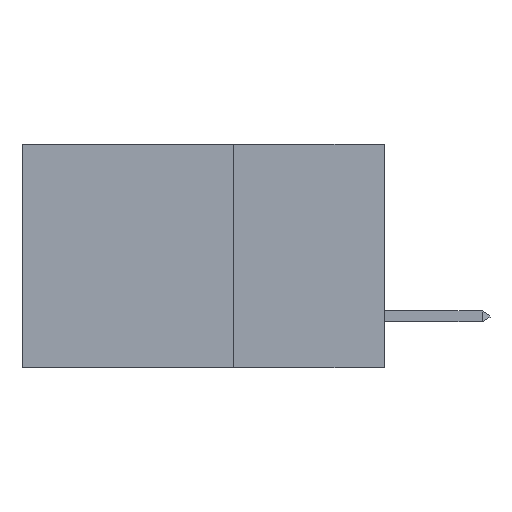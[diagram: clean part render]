
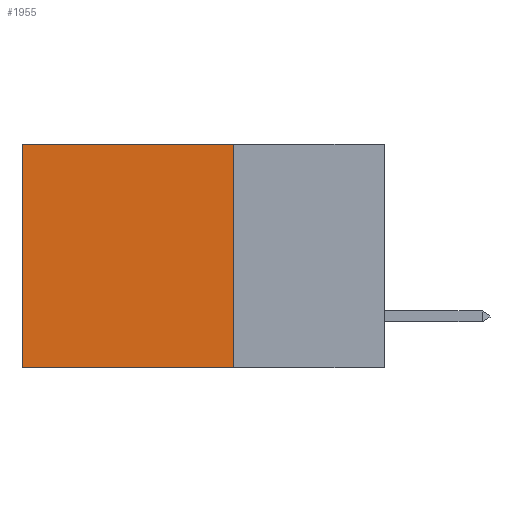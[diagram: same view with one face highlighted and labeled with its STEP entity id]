
A CAD part, left-side view. The second image highlights one B-rep face of the part: STEP entity #1955.
In plain terms, the highlighted planar face has unit normal (-1, 0, 0).
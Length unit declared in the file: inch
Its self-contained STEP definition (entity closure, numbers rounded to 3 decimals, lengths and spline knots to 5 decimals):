
#151 = VERTEX_POINT ( 'NONE', #10503 ) ;
#1612 = CARTESIAN_POINT ( 'NONE',  ( 0.2875, 0.6, 0. ) ) ;
#1689 = LINE ( 'NONE', #12362, #12950 ) ;
#1955 = ADVANCED_FACE ( 'NONE', ( #15050 ), #16464, .F. ) ;
#2047 = CARTESIAN_POINT ( 'NONE',  ( 0.2875, 0.25, -0.37 ) ) ;
#2986 = VERTEX_POINT ( 'NONE', #16378 ) ;
#3120 = DIRECTION ( 'NONE',  ( 0., 0., -1. ) ) ;
#3266 = VECTOR ( 'NONE', #13111, 39.37008 ) ;
#4010 = LINE ( 'NONE', #1612, #14661 ) ;
#4297 = EDGE_CURVE ( 'NONE', #151, #12354, #7303, .T. ) ;
#5060 = DIRECTION ( 'NONE',  ( 0., 1., 0. ) ) ;
#5773 = EDGE_LOOP ( 'NONE', ( #12469, #10964, #14122, #10629 ) ) ;
#6057 = CARTESIAN_POINT ( 'NONE',  ( 0.2875, 0.25, 0. ) ) ;
#7303 = LINE ( 'NONE', #15601, #3266 ) ;
#8840 = EDGE_CURVE ( 'NONE', #2986, #11443, #4010, .T. ) ;
#9416 = DIRECTION ( 'NONE',  ( 0., 0., -1. ) ) ;
#10264 = CARTESIAN_POINT ( 'NONE',  ( 0.2875, 0.6, -0.37 ) ) ;
#10347 = VECTOR ( 'NONE', #17449, 39.37008 ) ;
#10503 = CARTESIAN_POINT ( 'NONE',  ( 0.2875, 0.25, 0. ) ) ;
#10629 = ORIENTED_EDGE ( 'NONE', *, *, #16732, .T. ) ;
#10964 = ORIENTED_EDGE ( 'NONE', *, *, #13193, .F. ) ;
#11443 = VERTEX_POINT ( 'NONE', #10264 ) ;
#12354 = VERTEX_POINT ( 'NONE', #2047 ) ;
#12362 = CARTESIAN_POINT ( 'NONE',  ( 0.2875, 0.25, -0.37 ) ) ;
#12469 = ORIENTED_EDGE ( 'NONE', *, *, #8840, .T. ) ;
#12950 = VECTOR ( 'NONE', #5060, 39.37008 ) ;
#13111 = DIRECTION ( 'NONE',  ( 0., 0., -1. ) ) ;
#13193 = EDGE_CURVE ( 'NONE', #12354, #11443, #1689, .T. ) ;
#13976 = LINE ( 'NONE', #6057, #10347 ) ;
#14122 = ORIENTED_EDGE ( 'NONE', *, *, #4297, .F. ) ;
#14661 = VECTOR ( 'NONE', #3120, 39.37008 ) ;
#15050 = FACE_OUTER_BOUND ( 'NONE', #5773, .T. ) ;
#15601 = CARTESIAN_POINT ( 'NONE',  ( 0.2875, 0.25, 0. ) ) ;
#16378 = CARTESIAN_POINT ( 'NONE',  ( 0.2875, 0.6, 0. ) ) ;
#16464 = PLANE ( 'NONE',  #17403 ) ;
#16732 = EDGE_CURVE ( 'NONE', #151, #2986, #13976, .T. ) ;
#17403 = AXIS2_PLACEMENT_3D ( 'NONE', #18206, #18493, #9416 ) ;
#17449 = DIRECTION ( 'NONE',  ( 0., 1., 0. ) ) ;
#18206 = CARTESIAN_POINT ( 'NONE',  ( 0.2875, 0.25, 0. ) ) ;
#18493 = DIRECTION ( 'NONE',  ( 1., 0., 0. ) ) ;
